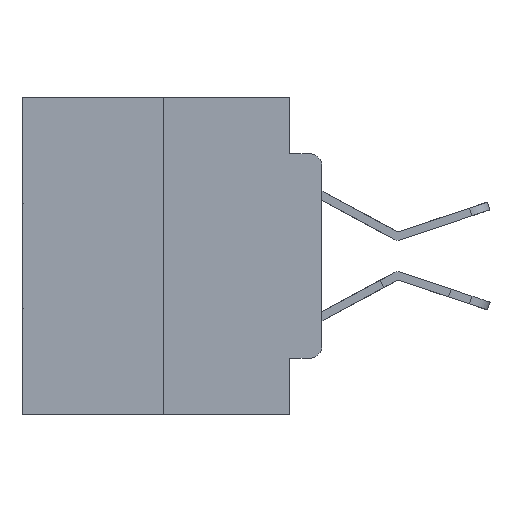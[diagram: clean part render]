
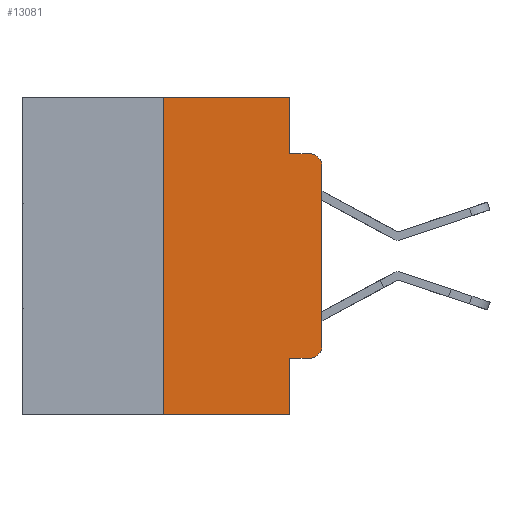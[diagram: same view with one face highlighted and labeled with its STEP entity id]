
A CAD part, left-side view. The second image highlights one B-rep face of the part: STEP entity #13081.
In plain terms, the highlighted planar face has unit normal (-1, 0, 0).
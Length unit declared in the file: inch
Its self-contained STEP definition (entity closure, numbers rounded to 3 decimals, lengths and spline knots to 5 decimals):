
#23 = EDGE_CURVE ( 'NONE', #16448, #9600, #14335, .T. ) ;
#113 = CARTESIAN_POINT ( 'NONE',  ( 0., 0.02, -0.1085 ) ) ;
#423 = AXIS2_PLACEMENT_3D ( 'NONE', #21846, #26500, #17749 ) ;
#1261 = VECTOR ( 'NONE', #25489, 39.37008 ) ;
#1484 = DIRECTION ( 'NONE',  ( 0., 0., 1. ) ) ;
#1680 = ORIENTED_EDGE ( 'NONE', *, *, #2380, .T. ) ;
#1984 = LINE ( 'NONE', #12840, #22782 ) ;
#2184 = VERTEX_POINT ( 'NONE', #27398 ) ;
#2197 = VERTEX_POINT ( 'NONE', #16496 ) ;
#2218 = CARTESIAN_POINT ( 'NONE',  ( 0., 0.051, -0.4115 ) ) ;
#2380 = EDGE_CURVE ( 'NONE', #19551, #24254, #6052, .T. ) ;
#2841 = LINE ( 'NONE', #9309, #15256 ) ;
#3435 = CARTESIAN_POINT ( 'NONE',  ( 0., 0.473, 0. ) ) ;
#3839 = LINE ( 'NONE', #16834, #1261 ) ;
#4237 = CARTESIAN_POINT ( 'NONE',  ( 0., 0.051, -0.0885 ) ) ;
#4642 = ORIENTED_EDGE ( 'NONE', *, *, #14664, .T. ) ;
#4685 = VECTOR ( 'NONE', #25554, 39.37008 ) ;
#4691 = CARTESIAN_POINT ( 'NONE',  ( 0., 0.051, -0.0885 ) ) ;
#5044 = LINE ( 'NONE', #7182, #10787 ) ;
#5818 = DIRECTION ( 'NONE',  ( 0., 0., -1. ) ) ;
#5956 = CARTESIAN_POINT ( 'NONE',  ( 0., 0., -0.1085 ) ) ;
#6052 = LINE ( 'NONE', #2218, #4685 ) ;
#6641 = ORIENTED_EDGE ( 'NONE', *, *, #19291, .T. ) ;
#7182 = CARTESIAN_POINT ( 'NONE',  ( 0., 0.25, 0. ) ) ;
#8130 = ORIENTED_EDGE ( 'NONE', *, *, #9154, .F. ) ;
#8581 = VERTEX_POINT ( 'NONE', #26661 ) ;
#8770 = DIRECTION ( 'NONE',  ( 0., 0., -1. ) ) ;
#9154 = EDGE_CURVE ( 'NONE', #2184, #27099, #3839, .T. ) ;
#9309 = CARTESIAN_POINT ( 'NONE',  ( 0., 0.473, -0.5 ) ) ;
#9600 = VERTEX_POINT ( 'NONE', #5956 ) ;
#9897 = DIRECTION ( 'NONE',  ( 0., 0., -1. ) ) ;
#10787 = VECTOR ( 'NONE', #11259, 39.37008 ) ;
#11011 = CARTESIAN_POINT ( 'NONE',  ( 0., 0.051, 0. ) ) ;
#11048 = ORIENTED_EDGE ( 'NONE', *, *, #17690, .F. ) ;
#11259 = DIRECTION ( 'NONE',  ( 0., 0., 1. ) ) ;
#11855 = LINE ( 'NONE', #16230, #16070 ) ;
#12255 = ORIENTED_EDGE ( 'NONE', *, *, #14931, .F. ) ;
#12840 = CARTESIAN_POINT ( 'NONE',  ( 0., 0.051, 0. ) ) ;
#13081 = ADVANCED_FACE ( 'NONE', ( #22925 ), #22787, .F. ) ;
#13308 = EDGE_CURVE ( 'NONE', #27099, #14253, #1984, .T. ) ;
#13588 = ORIENTED_EDGE ( 'NONE', *, *, #13308, .F. ) ;
#13701 = DIRECTION ( 'NONE',  ( 0., -1., 0. ) ) ;
#14253 = VERTEX_POINT ( 'NONE', #4691 ) ;
#14335 = LINE ( 'NONE', #22975, #22983 ) ;
#14664 = EDGE_CURVE ( 'NONE', #9600, #26572, #23744, .T. ) ;
#14931 = EDGE_CURVE ( 'NONE', #19551, #2197, #11855, .T. ) ;
#15256 = VECTOR ( 'NONE', #13701, 39.37008 ) ;
#15551 = CARTESIAN_POINT ( 'NONE',  ( 0., 0.02, -0.0885 ) ) ;
#15759 = CIRCLE ( 'NONE', #423, 0.02 ) ;
#15982 = AXIS2_PLACEMENT_3D ( 'NONE', #3435, #27168, #9897 ) ;
#16070 = VECTOR ( 'NONE', #5818, 39.37008 ) ;
#16189 = VECTOR ( 'NONE', #26146, 39.37008 ) ;
#16230 = CARTESIAN_POINT ( 'NONE',  ( 0., 0.051, 0. ) ) ;
#16448 = VERTEX_POINT ( 'NONE', #17929 ) ;
#16496 = CARTESIAN_POINT ( 'NONE',  ( 0., 0.051, -0.5 ) ) ;
#16834 = CARTESIAN_POINT ( 'NONE',  ( 0., 0.473, 0. ) ) ;
#17396 = CARTESIAN_POINT ( 'NONE',  ( 0., 0.02, -0.4115 ) ) ;
#17690 = EDGE_CURVE ( 'NONE', #14253, #26572, #25877, .T. ) ;
#17749 = DIRECTION ( 'NONE',  ( 0., 0., -1. ) ) ;
#17929 = CARTESIAN_POINT ( 'NONE',  ( 0., 0., -0.3915 ) ) ;
#19291 = EDGE_CURVE ( 'NONE', #8581, #2197, #2841, .T. ) ;
#19551 = VERTEX_POINT ( 'NONE', #21739 ) ;
#19678 = EDGE_CURVE ( 'NONE', #8581, #2184, #5044, .T. ) ;
#20151 = ORIENTED_EDGE ( 'NONE', *, *, #23, .T. ) ;
#20157 = EDGE_CURVE ( 'NONE', #24254, #16448, #15759, .T. ) ;
#21050 = AXIS2_PLACEMENT_3D ( 'NONE', #113, #23343, #8770 ) ;
#21739 = CARTESIAN_POINT ( 'NONE',  ( 0., 0.051, -0.4115 ) ) ;
#21846 = CARTESIAN_POINT ( 'NONE',  ( 0., 0.02, -0.3915 ) ) ;
#22782 = VECTOR ( 'NONE', #27847, 39.37008 ) ;
#22787 = PLANE ( 'NONE',  #15982 ) ;
#22925 = FACE_OUTER_BOUND ( 'NONE', #23754, .T. ) ;
#22975 = CARTESIAN_POINT ( 'NONE',  ( 0., 0., 0. ) ) ;
#22983 = VECTOR ( 'NONE', #1484, 39.37008 ) ;
#23343 = DIRECTION ( 'NONE',  ( -1., 0., 0. ) ) ;
#23744 = CIRCLE ( 'NONE', #21050, 0.02 ) ;
#23754 = EDGE_LOOP ( 'NONE', ( #20151, #4642, #11048, #13588, #8130, #25023, #6641, #12255, #1680, #25959 ) ) ;
#24254 = VERTEX_POINT ( 'NONE', #17396 ) ;
#25023 = ORIENTED_EDGE ( 'NONE', *, *, #19678, .F. ) ;
#25489 = DIRECTION ( 'NONE',  ( 0., -1., 0. ) ) ;
#25554 = DIRECTION ( 'NONE',  ( 0., -1., 0. ) ) ;
#25877 = LINE ( 'NONE', #4237, #16189 ) ;
#25959 = ORIENTED_EDGE ( 'NONE', *, *, #20157, .T. ) ;
#26146 = DIRECTION ( 'NONE',  ( 0., -1., 0. ) ) ;
#26500 = DIRECTION ( 'NONE',  ( -1., 0., 0. ) ) ;
#26572 = VERTEX_POINT ( 'NONE', #15551 ) ;
#26661 = CARTESIAN_POINT ( 'NONE',  ( 0., 0.25, -0.5 ) ) ;
#27099 = VERTEX_POINT ( 'NONE', #11011 ) ;
#27168 = DIRECTION ( 'NONE',  ( 1., 0., 0. ) ) ;
#27398 = CARTESIAN_POINT ( 'NONE',  ( 0., 0.25, 0. ) ) ;
#27847 = DIRECTION ( 'NONE',  ( 0., 0., -1. ) ) ;
